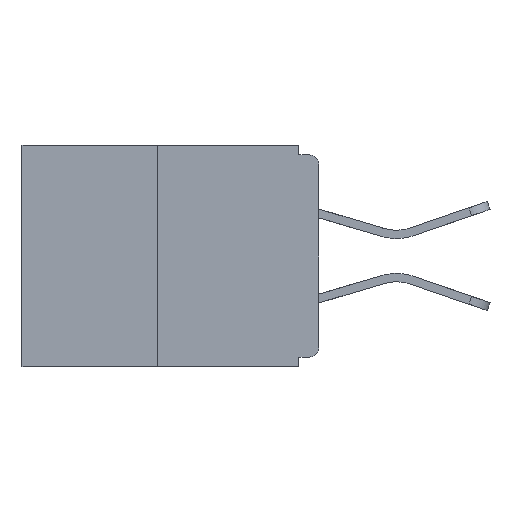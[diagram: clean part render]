
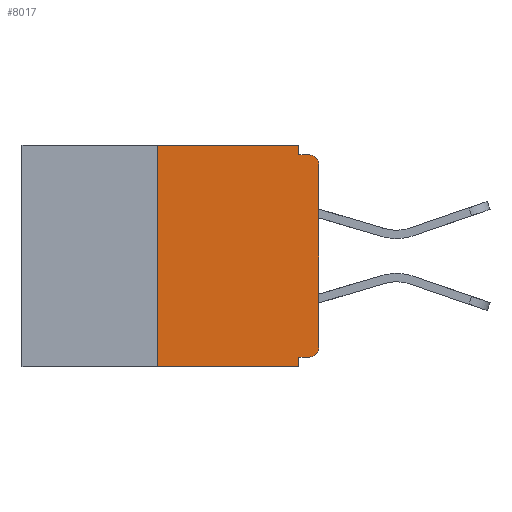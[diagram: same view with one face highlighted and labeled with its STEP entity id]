
A CAD part, left-side view. The second image highlights one B-rep face of the part: STEP entity #8017.
In plain terms, the highlighted planar face has unit normal (-1, 0, 0).
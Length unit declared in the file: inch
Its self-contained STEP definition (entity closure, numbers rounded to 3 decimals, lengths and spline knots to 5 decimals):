
#224 = CARTESIAN_POINT ( 'NONE',  ( 0., 0.25, 0. ) ) ;
#362 = CARTESIAN_POINT ( 'NONE',  ( 0., 0.031, 0. ) ) ;
#523 = VERTEX_POINT ( 'NONE', #224 ) ;
#600 = VERTEX_POINT ( 'NONE', #11919 ) ;
#671 = VERTEX_POINT ( 'NONE', #362 ) ;
#824 = CARTESIAN_POINT ( 'NONE',  ( 0., 0.25, 0. ) ) ;
#921 = CARTESIAN_POINT ( 'NONE',  ( 0., 0.46, 0. ) ) ;
#1028 = CARTESIAN_POINT ( 'NONE',  ( 0., 0., 0. ) ) ;
#1076 = ORIENTED_EDGE ( 'NONE', *, *, #10052, .F. ) ;
#1077 = DIRECTION ( 'NONE',  ( 0., 0., -1. ) ) ;
#1092 = EDGE_LOOP ( 'NONE', ( #11728, #1541, #11767, #5570, #8813, #2978, #5247, #1247, #1076, #10846 ) ) ;
#1247 = ORIENTED_EDGE ( 'NONE', *, *, #8780, .T. ) ;
#1334 = CARTESIAN_POINT ( 'NONE',  ( 0., 0., -0.03 ) ) ;
#1539 = CARTESIAN_POINT ( 'NONE',  ( 0., 0.031, -0.015 ) ) ;
#1541 = ORIENTED_EDGE ( 'NONE', *, *, #12305, .F. ) ;
#1785 = DIRECTION ( 'NONE',  ( 0., 1., 0. ) ) ;
#1854 = AXIS2_PLACEMENT_3D ( 'NONE', #9756, #2023, #6787 ) ;
#1935 = CARTESIAN_POINT ( 'NONE',  ( 0., 0.25, -0.343 ) ) ;
#2018 = VECTOR ( 'NONE', #4111, 39.37008 ) ;
#2023 = DIRECTION ( 'NONE',  ( -1., 0., 0. ) ) ;
#2370 = VECTOR ( 'NONE', #5760, 39.37008 ) ;
#2449 = EDGE_CURVE ( 'NONE', #523, #671, #7921, .T. ) ;
#2477 = CIRCLE ( 'NONE', #1854, 0.015 ) ;
#2481 = LINE ( 'NONE', #11410, #3090 ) ;
#2660 = PLANE ( 'NONE',  #7762 ) ;
#2808 = LINE ( 'NONE', #824, #2370 ) ;
#2831 = CARTESIAN_POINT ( 'NONE',  ( 0., 0.031, -0.328 ) ) ;
#2912 = CARTESIAN_POINT ( 'NONE',  ( 0., 0.46, -0.343 ) ) ;
#2941 = VECTOR ( 'NONE', #5789, 39.37008 ) ;
#2978 = ORIENTED_EDGE ( 'NONE', *, *, #3622, .T. ) ;
#3057 = CIRCLE ( 'NONE', #7438, 0.015 ) ;
#3090 = VECTOR ( 'NONE', #3663, 39.37008 ) ;
#3253 = EDGE_CURVE ( 'NONE', #10290, #3331, #12253, .T. ) ;
#3326 = EDGE_CURVE ( 'NONE', #3892, #8150, #11059, .T. ) ;
#3331 = VERTEX_POINT ( 'NONE', #9827 ) ;
#3378 = DIRECTION ( 'NONE',  ( 0., 0., -1. ) ) ;
#3405 = DIRECTION ( 'NONE',  ( 1., 0., 0. ) ) ;
#3622 = EDGE_CURVE ( 'NONE', #11982, #3892, #2477, .T. ) ;
#3663 = DIRECTION ( 'NONE',  ( 0., 0., -1. ) ) ;
#3892 = VERTEX_POINT ( 'NONE', #5728 ) ;
#3957 = VECTOR ( 'NONE', #3378, 39.37008 ) ;
#4111 = DIRECTION ( 'NONE',  ( 0., 0., 1. ) ) ;
#4375 = CARTESIAN_POINT ( 'NONE',  ( 0., 0.015, -0.328 ) ) ;
#5247 = ORIENTED_EDGE ( 'NONE', *, *, #3326, .T. ) ;
#5570 = ORIENTED_EDGE ( 'NONE', *, *, #7949, .F. ) ;
#5687 = VECTOR ( 'NONE', #11467, 39.37008 ) ;
#5728 = CARTESIAN_POINT ( 'NONE',  ( 0., 0., -0.313 ) ) ;
#5760 = DIRECTION ( 'NONE',  ( 0., 0., 1. ) ) ;
#5789 = DIRECTION ( 'NONE',  ( 0., -1., 0. ) ) ;
#6266 = CARTESIAN_POINT ( 'NONE',  ( 0., 0.031, -0.343 ) ) ;
#6738 = DIRECTION ( 'NONE',  ( -1., 0., 0. ) ) ;
#6787 = DIRECTION ( 'NONE',  ( 0., 0., -1. ) ) ;
#7075 = DIRECTION ( 'NONE',  ( 0., 0., -1. ) ) ;
#7178 = VECTOR ( 'NONE', #1785, 39.37008 ) ;
#7342 = EDGE_CURVE ( 'NONE', #671, #9845, #2481, .T. ) ;
#7438 = AXIS2_PLACEMENT_3D ( 'NONE', #10629, #6738, #1077 ) ;
#7762 = AXIS2_PLACEMENT_3D ( 'NONE', #10318, #3405, #7075 ) ;
#7921 = LINE ( 'NONE', #921, #5687 ) ;
#7949 = EDGE_CURVE ( 'NONE', #8055, #3331, #11959, .T. ) ;
#7973 = CARTESIAN_POINT ( 'NONE',  ( 0., 0., -0.015 ) ) ;
#8017 = ADVANCED_FACE ( 'NONE', ( #8021 ), #2660, .F. ) ;
#8021 = FACE_OUTER_BOUND ( 'NONE', #1092, .T. ) ;
#8055 = VERTEX_POINT ( 'NONE', #2831 ) ;
#8150 = VERTEX_POINT ( 'NONE', #1334 ) ;
#8710 = LINE ( 'NONE', #7973, #8863 ) ;
#8780 = EDGE_CURVE ( 'NONE', #8150, #600, #3057, .T. ) ;
#8813 = ORIENTED_EDGE ( 'NONE', *, *, #12298, .F. ) ;
#8863 = VECTOR ( 'NONE', #10968, 39.37008 ) ;
#9066 = CARTESIAN_POINT ( 'NONE',  ( 0., 0., -0.328 ) ) ;
#9756 = CARTESIAN_POINT ( 'NONE',  ( 0., 0.015, -0.313 ) ) ;
#9827 = CARTESIAN_POINT ( 'NONE',  ( 0., 0.031, -0.343 ) ) ;
#9845 = VERTEX_POINT ( 'NONE', #1539 ) ;
#10052 = EDGE_CURVE ( 'NONE', #9845, #600, #8710, .T. ) ;
#10139 = LINE ( 'NONE', #9066, #7178 ) ;
#10290 = VERTEX_POINT ( 'NONE', #1935 ) ;
#10318 = CARTESIAN_POINT ( 'NONE',  ( 0., 0.46, 0. ) ) ;
#10629 = CARTESIAN_POINT ( 'NONE',  ( 0., 0.015, -0.03 ) ) ;
#10846 = ORIENTED_EDGE ( 'NONE', *, *, #7342, .F. ) ;
#10968 = DIRECTION ( 'NONE',  ( 0., -1., 0. ) ) ;
#11059 = LINE ( 'NONE', #1028, #2018 ) ;
#11410 = CARTESIAN_POINT ( 'NONE',  ( 0., 0.031, 0. ) ) ;
#11467 = DIRECTION ( 'NONE',  ( 0., -1., 0. ) ) ;
#11728 = ORIENTED_EDGE ( 'NONE', *, *, #2449, .F. ) ;
#11767 = ORIENTED_EDGE ( 'NONE', *, *, #3253, .T. ) ;
#11919 = CARTESIAN_POINT ( 'NONE',  ( 0., 0.015, -0.015 ) ) ;
#11959 = LINE ( 'NONE', #6266, #3957 ) ;
#11982 = VERTEX_POINT ( 'NONE', #4375 ) ;
#12253 = LINE ( 'NONE', #2912, #2941 ) ;
#12298 = EDGE_CURVE ( 'NONE', #11982, #8055, #10139, .T. ) ;
#12305 = EDGE_CURVE ( 'NONE', #10290, #523, #2808, .T. ) ;
